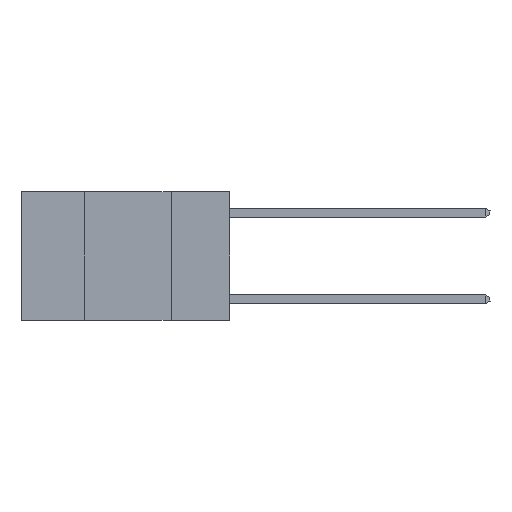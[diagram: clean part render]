
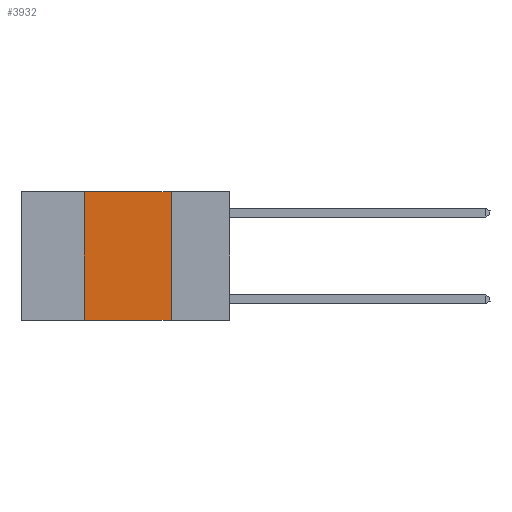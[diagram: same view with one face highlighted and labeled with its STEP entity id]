
A CAD part, left-side view. The second image highlights one B-rep face of the part: STEP entity #3932.
In plain terms, the highlighted planar face has unit normal (-1, 0, 0).
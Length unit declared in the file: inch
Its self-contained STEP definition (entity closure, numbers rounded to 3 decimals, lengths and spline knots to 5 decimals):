
#162 = AXIS2_PLACEMENT_3D ( 'NONE', #12228, #5655, #196 ) ;
#196 = DIRECTION ( 'NONE',  ( 0., 0., -1. ) ) ;
#814 = EDGE_CURVE ( 'NONE', #14852, #16956, #16960, .T. ) ;
#956 = VECTOR ( 'NONE', #3877, 39.37008 ) ;
#2199 = CARTESIAN_POINT ( 'NONE',  ( 0., 0.17, 0. ) ) ;
#2812 = ORIENTED_EDGE ( 'NONE', *, *, #814, .F. ) ;
#3877 = DIRECTION ( 'NONE',  ( 0., 0., 1. ) ) ;
#3908 = DIRECTION ( 'NONE',  ( 0., 0., -1. ) ) ;
#3932 = ADVANCED_FACE ( 'NONE', ( #4281 ), #4444, .F. ) ;
#4281 = FACE_OUTER_BOUND ( 'NONE', #12567, .T. ) ;
#4444 = PLANE ( 'NONE',  #162 ) ;
#4555 = DIRECTION ( 'NONE',  ( 0., -1., 0. ) ) ;
#4842 = ORIENTED_EDGE ( 'NONE', *, *, #8804, .T. ) ;
#5655 = DIRECTION ( 'NONE',  ( 1., 0., 0. ) ) ;
#5846 = LINE ( 'NONE', #11101, #13549 ) ;
#6509 = EDGE_CURVE ( 'NONE', #7819, #14852, #15581, .T. ) ;
#7722 = CARTESIAN_POINT ( 'NONE',  ( 0., 0.42, 0. ) ) ;
#7819 = VERTEX_POINT ( 'NONE', #17105 ) ;
#7928 = CARTESIAN_POINT ( 'NONE',  ( 0., 0.42, 0. ) ) ;
#8804 = EDGE_CURVE ( 'NONE', #7819, #15262, #5846, .T. ) ;
#8887 = VECTOR ( 'NONE', #14256, 39.37008 ) ;
#10423 = CARTESIAN_POINT ( 'NONE',  ( 0., 0.6, 0. ) ) ;
#10459 = CARTESIAN_POINT ( 'NONE',  ( 0., 0.17, 0. ) ) ;
#11101 = CARTESIAN_POINT ( 'NONE',  ( 0., 0.6, -0.37 ) ) ;
#12191 = LINE ( 'NONE', #10459, #14243 ) ;
#12228 = CARTESIAN_POINT ( 'NONE',  ( 0., 0.6, 0. ) ) ;
#12567 = EDGE_LOOP ( 'NONE', ( #14991, #2812, #15633, #4842 ) ) ;
#13549 = VECTOR ( 'NONE', #4555, 39.37008 ) ;
#14209 = CARTESIAN_POINT ( 'NONE',  ( 0., 0.17, -0.37 ) ) ;
#14243 = VECTOR ( 'NONE', #3908, 39.37008 ) ;
#14256 = DIRECTION ( 'NONE',  ( 0., -1., 0. ) ) ;
#14852 = VERTEX_POINT ( 'NONE', #7722 ) ;
#14991 = ORIENTED_EDGE ( 'NONE', *, *, #15465, .F. ) ;
#15262 = VERTEX_POINT ( 'NONE', #14209 ) ;
#15465 = EDGE_CURVE ( 'NONE', #16956, #15262, #12191, .T. ) ;
#15581 = LINE ( 'NONE', #7928, #956 ) ;
#15633 = ORIENTED_EDGE ( 'NONE', *, *, #6509, .F. ) ;
#16956 = VERTEX_POINT ( 'NONE', #2199 ) ;
#16960 = LINE ( 'NONE', #10423, #8887 ) ;
#17105 = CARTESIAN_POINT ( 'NONE',  ( 0., 0.42, -0.37 ) ) ;
